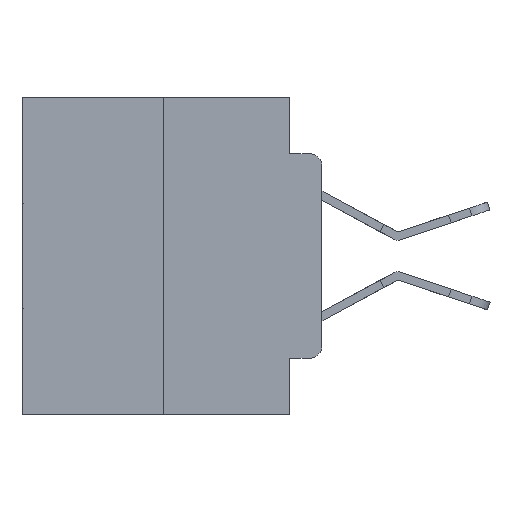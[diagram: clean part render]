
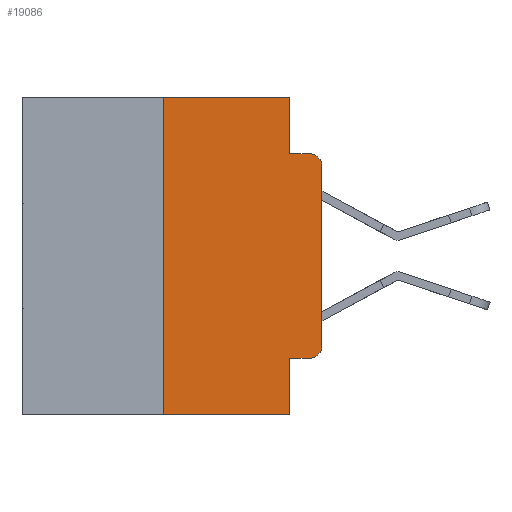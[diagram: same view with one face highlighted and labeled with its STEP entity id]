
A CAD part, left-side view. The second image highlights one B-rep face of the part: STEP entity #19086.
In plain terms, the highlighted planar face has unit normal (-1, 0, 0).
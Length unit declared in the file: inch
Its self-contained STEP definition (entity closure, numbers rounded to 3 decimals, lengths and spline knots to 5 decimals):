
#840 = LINE ( 'NONE', #15575, #21205 ) ;
#1158 = VECTOR ( 'NONE', #10538, 39.37008 ) ;
#1876 = CARTESIAN_POINT ( 'NONE',  ( 0., 0.25, -0.5 ) ) ;
#2202 = EDGE_CURVE ( 'NONE', #28840, #3686, #9733, .T. ) ;
#2335 = CARTESIAN_POINT ( 'NONE',  ( 0., 0.02, -0.3915 ) ) ;
#2663 = DIRECTION ( 'NONE',  ( 0., 0., 1. ) ) ;
#2703 = LINE ( 'NONE', #22055, #12509 ) ;
#3092 = VERTEX_POINT ( 'NONE', #13506 ) ;
#3686 = VERTEX_POINT ( 'NONE', #9189 ) ;
#3721 = CARTESIAN_POINT ( 'NONE',  ( 0., 0.473, 0. ) ) ;
#3818 = ORIENTED_EDGE ( 'NONE', *, *, #24573, .F. ) ;
#4027 = CIRCLE ( 'NONE', #22754, 0.02 ) ;
#4240 = VERTEX_POINT ( 'NONE', #1876 ) ;
#5150 = CARTESIAN_POINT ( 'NONE',  ( 0., 0.473, 0. ) ) ;
#5908 = DIRECTION ( 'NONE',  ( 0., 0., -1. ) ) ;
#6009 = CARTESIAN_POINT ( 'NONE',  ( 0., 0.25, 0. ) ) ;
#6368 = VECTOR ( 'NONE', #25639, 39.37008 ) ;
#6451 = CARTESIAN_POINT ( 'NONE',  ( 0., 0.02, -0.1085 ) ) ;
#6645 = DIRECTION ( 'NONE',  ( -1., 0., 0. ) ) ;
#7227 = DIRECTION ( 'NONE',  ( 0., -1., 0. ) ) ;
#7306 = VERTEX_POINT ( 'NONE', #22285 ) ;
#8147 = PLANE ( 'NONE',  #21194 ) ;
#8278 = EDGE_CURVE ( 'NONE', #14169, #18691, #20931, .T. ) ;
#8310 = DIRECTION ( 'NONE',  ( 0., 0., -1. ) ) ;
#8578 = CARTESIAN_POINT ( 'NONE',  ( 0., 0.051, -0.4115 ) ) ;
#8595 = DIRECTION ( 'NONE',  ( 0., -1., 0. ) ) ;
#8639 = EDGE_CURVE ( 'NONE', #18691, #12946, #4027, .T. ) ;
#9189 = CARTESIAN_POINT ( 'NONE',  ( 0., 0.051, -0.5 ) ) ;
#9324 = VERTEX_POINT ( 'NONE', #27284 ) ;
#9643 = CARTESIAN_POINT ( 'NONE',  ( 0., 0., 0. ) ) ;
#9720 = EDGE_CURVE ( 'NONE', #4240, #9324, #13069, .T. ) ;
#9733 = LINE ( 'NONE', #19397, #28040 ) ;
#10538 = DIRECTION ( 'NONE',  ( 0., 0., 1. ) ) ;
#10605 = DIRECTION ( 'NONE',  ( 0., 0., -1. ) ) ;
#11140 = VERTEX_POINT ( 'NONE', #28872 ) ;
#12029 = CARTESIAN_POINT ( 'NONE',  ( 0., 0.473, -0.5 ) ) ;
#12036 = ORIENTED_EDGE ( 'NONE', *, *, #24126, .F. ) ;
#12230 = ORIENTED_EDGE ( 'NONE', *, *, #8278, .T. ) ;
#12509 = VECTOR ( 'NONE', #8595, 39.37008 ) ;
#12946 = VERTEX_POINT ( 'NONE', #17222 ) ;
#13069 = LINE ( 'NONE', #6009, #1158 ) ;
#13506 = CARTESIAN_POINT ( 'NONE',  ( 0., 0.02, -0.4115 ) ) ;
#14150 = ORIENTED_EDGE ( 'NONE', *, *, #20785, .T. ) ;
#14169 = VERTEX_POINT ( 'NONE', #19046 ) ;
#14545 = ORIENTED_EDGE ( 'NONE', *, *, #19820, .T. ) ;
#15002 = LINE ( 'NONE', #5150, #23462 ) ;
#15575 = CARTESIAN_POINT ( 'NONE',  ( 0., 0.051, -0.4115 ) ) ;
#16325 = EDGE_LOOP ( 'NONE', ( #12230, #17463, #3818, #21953, #12036, #18617, #14150, #24018, #14545, #21209 ) ) ;
#17222 = CARTESIAN_POINT ( 'NONE',  ( 0., 0.02, -0.0885 ) ) ;
#17372 = VECTOR ( 'NONE', #8310, 39.37008 ) ;
#17422 = VECTOR ( 'NONE', #2663, 39.37008 ) ;
#17463 = ORIENTED_EDGE ( 'NONE', *, *, #8639, .T. ) ;
#18617 = ORIENTED_EDGE ( 'NONE', *, *, #9720, .F. ) ;
#18691 = VERTEX_POINT ( 'NONE', #29037 ) ;
#18834 = AXIS2_PLACEMENT_3D ( 'NONE', #2335, #6645, #20327 ) ;
#19046 = CARTESIAN_POINT ( 'NONE',  ( 0., 0., -0.3915 ) ) ;
#19086 = ADVANCED_FACE ( 'NONE', ( #28683 ), #8147, .F. ) ;
#19397 = CARTESIAN_POINT ( 'NONE',  ( 0., 0.051, 0. ) ) ;
#19763 = LINE ( 'NONE', #12029, #6368 ) ;
#19820 = EDGE_CURVE ( 'NONE', #28840, #3092, #840, .T. ) ;
#20327 = DIRECTION ( 'NONE',  ( 0., 0., -1. ) ) ;
#20785 = EDGE_CURVE ( 'NONE', #4240, #3686, #19763, .T. ) ;
#20931 = LINE ( 'NONE', #9643, #17422 ) ;
#21194 = AXIS2_PLACEMENT_3D ( 'NONE', #3721, #21816, #10605 ) ;
#21205 = VECTOR ( 'NONE', #22178, 39.37008 ) ;
#21209 = ORIENTED_EDGE ( 'NONE', *, *, #23976, .T. ) ;
#21816 = DIRECTION ( 'NONE',  ( 1., 0., 0. ) ) ;
#21953 = ORIENTED_EDGE ( 'NONE', *, *, #26121, .F. ) ;
#22055 = CARTESIAN_POINT ( 'NONE',  ( 0., 0.051, -0.0885 ) ) ;
#22088 = DIRECTION ( 'NONE',  ( -1., 0., 0. ) ) ;
#22178 = DIRECTION ( 'NONE',  ( 0., -1., 0. ) ) ;
#22285 = CARTESIAN_POINT ( 'NONE',  ( 0., 0.051, -0.0885 ) ) ;
#22306 = LINE ( 'NONE', #26303, #17372 ) ;
#22754 = AXIS2_PLACEMENT_3D ( 'NONE', #6451, #22088, #29094 ) ;
#23462 = VECTOR ( 'NONE', #7227, 39.37008 ) ;
#23976 = EDGE_CURVE ( 'NONE', #3092, #14169, #27655, .T. ) ;
#24018 = ORIENTED_EDGE ( 'NONE', *, *, #2202, .F. ) ;
#24126 = EDGE_CURVE ( 'NONE', #9324, #11140, #15002, .T. ) ;
#24573 = EDGE_CURVE ( 'NONE', #7306, #12946, #2703, .T. ) ;
#25639 = DIRECTION ( 'NONE',  ( 0., -1., 0. ) ) ;
#26121 = EDGE_CURVE ( 'NONE', #11140, #7306, #22306, .T. ) ;
#26303 = CARTESIAN_POINT ( 'NONE',  ( 0., 0.051, 0. ) ) ;
#27284 = CARTESIAN_POINT ( 'NONE',  ( 0., 0.25, 0. ) ) ;
#27655 = CIRCLE ( 'NONE', #18834, 0.02 ) ;
#28040 = VECTOR ( 'NONE', #5908, 39.37008 ) ;
#28683 = FACE_OUTER_BOUND ( 'NONE', #16325, .T. ) ;
#28840 = VERTEX_POINT ( 'NONE', #8578 ) ;
#28872 = CARTESIAN_POINT ( 'NONE',  ( 0., 0.051, 0. ) ) ;
#29037 = CARTESIAN_POINT ( 'NONE',  ( 0., 0., -0.1085 ) ) ;
#29094 = DIRECTION ( 'NONE',  ( 0., 0., -1. ) ) ;
